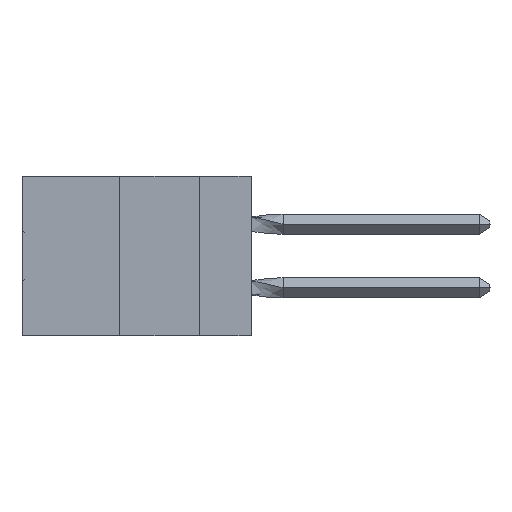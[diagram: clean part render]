
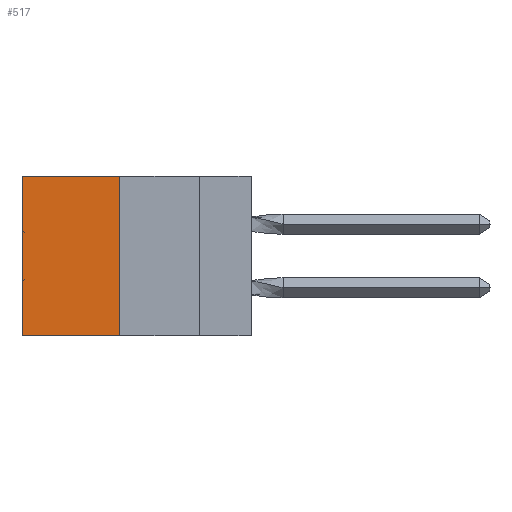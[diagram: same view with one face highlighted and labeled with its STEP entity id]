
A CAD part, left-side view. The second image highlights one B-rep face of the part: STEP entity #517.
In plain terms, the highlighted planar face has unit normal (-1, 0, 0).
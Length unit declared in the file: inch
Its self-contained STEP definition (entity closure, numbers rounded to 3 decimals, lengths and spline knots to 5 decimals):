
#517 = ADVANCED_FACE ( 'NONE', ( #34506 ), #10022, .F. ) ;
#1990 = DIRECTION ( 'NONE',  ( 0., 0., -1. ) ) ;
#2358 = VERTEX_POINT ( 'NONE', #42723 ) ;
#2871 = DIRECTION ( 'NONE',  ( 0., 0., -1. ) ) ;
#2876 = ORIENTED_EDGE ( 'NONE', *, *, #5231, .T. ) ;
#4069 = EDGE_LOOP ( 'NONE', ( #32823, #31338, #24508, #2876 ) ) ;
#4521 = CARTESIAN_POINT ( 'NONE',  ( 0.305, 0.413, -0.5 ) ) ;
#5231 = EDGE_CURVE ( 'NONE', #40488, #24253, #27700, .T. ) ;
#6603 = DIRECTION ( 'NONE',  ( 0., 0., -1. ) ) ;
#7163 = VECTOR ( 'NONE', #33419, 39.37008 ) ;
#7783 = CARTESIAN_POINT ( 'NONE',  ( 0.305, 0.72, 0. ) ) ;
#8362 = EDGE_CURVE ( 'NONE', #40488, #34710, #37777, .T. ) ;
#9398 = CARTESIAN_POINT ( 'NONE',  ( 0.305, 0.413, 0. ) ) ;
#9666 = VECTOR ( 'NONE', #6603, 39.37008 ) ;
#9829 = LINE ( 'NONE', #22017, #12975 ) ;
#10022 = PLANE ( 'NONE',  #16891 ) ;
#12975 = VECTOR ( 'NONE', #29812, 39.37008 ) ;
#16891 = AXIS2_PLACEMENT_3D ( 'NONE', #17886, #49668, #1990 ) ;
#17886 = CARTESIAN_POINT ( 'NONE',  ( 0.305, 0.413, -0.5 ) ) ;
#22017 = CARTESIAN_POINT ( 'NONE',  ( 0.305, 0.413, -0.5 ) ) ;
#24253 = VERTEX_POINT ( 'NONE', #7783 ) ;
#24508 = ORIENTED_EDGE ( 'NONE', *, *, #8362, .F. ) ;
#26757 = CARTESIAN_POINT ( 'NONE',  ( 0.305, 0.72, -0.5 ) ) ;
#27700 = LINE ( 'NONE', #9398, #7163 ) ;
#29812 = DIRECTION ( 'NONE',  ( 0., 1., 0. ) ) ;
#31338 = ORIENTED_EDGE ( 'NONE', *, *, #46218, .F. ) ;
#32435 = CARTESIAN_POINT ( 'NONE',  ( 0.305, 0.413, 0. ) ) ;
#32823 = ORIENTED_EDGE ( 'NONE', *, *, #35545, .T. ) ;
#33399 = LINE ( 'NONE', #26757, #40386 ) ;
#33419 = DIRECTION ( 'NONE',  ( 0., 1., 0. ) ) ;
#34506 = FACE_OUTER_BOUND ( 'NONE', #4069, .T. ) ;
#34710 = VERTEX_POINT ( 'NONE', #4521 ) ;
#35545 = EDGE_CURVE ( 'NONE', #24253, #2358, #33399, .T. ) ;
#37777 = LINE ( 'NONE', #38224, #9666 ) ;
#38224 = CARTESIAN_POINT ( 'NONE',  ( 0.305, 0.413, -0.5 ) ) ;
#40386 = VECTOR ( 'NONE', #2871, 39.37008 ) ;
#40488 = VERTEX_POINT ( 'NONE', #32435 ) ;
#42723 = CARTESIAN_POINT ( 'NONE',  ( 0.305, 0.72, -0.5 ) ) ;
#46218 = EDGE_CURVE ( 'NONE', #34710, #2358, #9829, .T. ) ;
#49668 = DIRECTION ( 'NONE',  ( 1., 0., 0. ) ) ;
